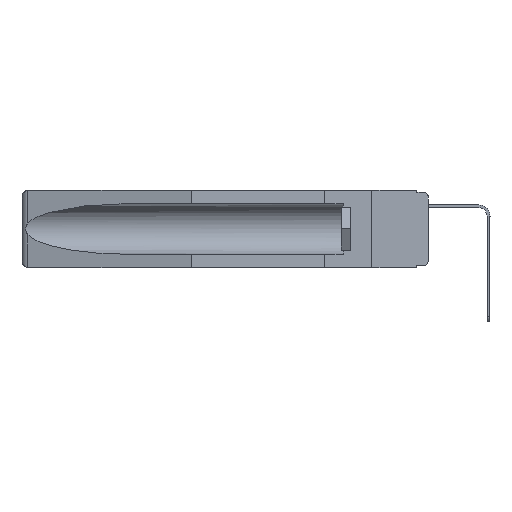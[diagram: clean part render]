
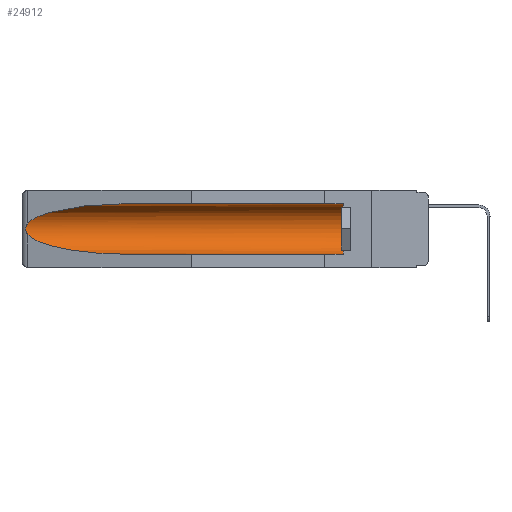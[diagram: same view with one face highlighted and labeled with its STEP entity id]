
A CAD part, left-side view. The second image highlights one B-rep face of the part: STEP entity #24912.
In plain terms, the highlighted cylindrical face has radius 2.857 mm (diameter 5.715 mm), a partial arc.
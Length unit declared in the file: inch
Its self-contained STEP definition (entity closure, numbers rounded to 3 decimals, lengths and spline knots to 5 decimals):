
#73 = CARTESIAN_POINT ( 'NONE',  ( 0.155, -0.30754, -0.059 ) ) ;
#210 = ORIENTED_EDGE ( 'NONE', *, *, #16794, .T. ) ;
#627 = VERTEX_POINT ( 'NONE', #7582 ) ;
#863 = EDGE_CURVE ( 'NONE', #627, #16626, #7154, .T. ) ;
#2396 = VERTEX_POINT ( 'NONE', #21390 ) ;
#2534 = EDGE_CURVE ( 'NONE', #627, #20455, #9218, .T. ) ;
#2753 = CARTESIAN_POINT ( 'NONE',  ( 0.2675, 1.53308, -0.17534 ) ) ;
#2929 = CARTESIAN_POINT ( 'NONE',  ( 0.155, 1.07973, -0.284 ) ) ;
#3039 = AXIS2_PLACEMENT_3D ( 'NONE', #8052, #11951, #4385 ) ;
#4385 = DIRECTION ( 'NONE',  ( 0., 0., 1. ) ) ;
#4728 = CARTESIAN_POINT ( 'NONE',  ( 0.26537, 1.52718, -0.14972 ) ) ;
#4890 = ORIENTED_EDGE ( 'NONE', *, *, #9705, .T. ) ;
#4946 = CYLINDRICAL_SURFACE ( 'NONE', #3039, 0.1125 ) ;
#5270 = VECTOR ( 'NONE', #25312, 39.37008 ) ;
#5434 = CARTESIAN_POINT ( 'NONE',  ( 0.155, 1.07973, -0.059 ) ) ;
#7154 = CIRCLE ( 'NONE', #8418, 0.1125 ) ;
#7582 = CARTESIAN_POINT ( 'NONE',  ( 0.155, 0.126, -0.284 ) ) ;
#8052 = CARTESIAN_POINT ( 'NONE',  ( 0.155, -0.30754, -0.1715 ) ) ;
#8418 = AXIS2_PLACEMENT_3D ( 'NONE', #24604, #16175, #23609 ) ;
#8905 = CARTESIAN_POINT ( 'NONE',  ( 0.21114, 1.30732, -0.284 ) ) ;
#9218 = LINE ( 'NONE', #10142, #16315 ) ;
#9551 = VERTEX_POINT ( 'NONE', #17956 ) ;
#9705 = EDGE_CURVE ( 'NONE', #9551, #20455, #12504, .T. ) ;
#10142 = CARTESIAN_POINT ( 'NONE',  ( 0.155, -0.30754, -0.284 ) ) ;
#10208 = CARTESIAN_POINT ( 'NONE',  ( 0.26597, 1.52961, -0.15275 ) ) ;
#10494 = LINE ( 'NONE', #73, #5270 ) ;
#10935 = ORIENTED_EDGE ( 'NONE', *, *, #23607, .T. ) ;
#11814 = DIRECTION ( 'NONE',  ( 0., 1., 0. ) ) ;
#11951 = DIRECTION ( 'NONE',  ( 0., 1., 0. ) ) ;
#12220 = EDGE_LOOP ( 'NONE', ( #10935, #210, #4890, #18144, #12949, #17336 ) ) ;
#12287 = CARTESIAN_POINT ( 'NONE',  ( 0.2673, 1.53269, -0.17917 ) ) ;
#12504 =( BOUNDED_CURVE ( )  B_SPLINE_CURVE ( 3, ( #22294, #20497, #8905, #2929 ),
 .UNSPECIFIED., .F., .F. ) 
 B_SPLINE_CURVE_WITH_KNOTS ( ( 4, 4 ),
 ( 0.1948, 1.5708 ),
 .UNSPECIFIED. ) 
 CURVE ( )  GEOMETRIC_REPRESENTATION_ITEM ( )  RATIONAL_B_SPLINE_CURVE ( ( 1., 0.848, 0.848, 1. ) ) 
 REPRESENTATION_ITEM ( '' )  );
#12949 = ORIENTED_EDGE ( 'NONE', *, *, #863, .T. ) ;
#13445 =( BOUNDED_CURVE ( )  B_SPLINE_CURVE ( 3, ( #5434, #17284, #23088, #23007 ),
 .UNSPECIFIED., .F., .T. ) 
 B_SPLINE_CURVE_WITH_KNOTS ( ( 4, 4 ),
 ( 4.71239, 6.08839 ),
 .UNSPECIFIED. ) 
 CURVE ( )  GEOMETRIC_REPRESENTATION_ITEM ( )  RATIONAL_B_SPLINE_CURVE ( ( 1., 0.848, 0.848, 1. ) ) 
 REPRESENTATION_ITEM ( '' )  );
#13766 = CARTESIAN_POINT ( 'NONE',  ( 0.155, 1.07973, -0.284 ) ) ;
#14045 = EDGE_CURVE ( 'NONE', #16626, #2396, #10494, .T. ) ;
#14366 = CARTESIAN_POINT ( 'NONE',  ( 0.2673, 1.5327, -0.16383 ) ) ;
#14525 = CARTESIAN_POINT ( 'NONE',  ( 0.26654, 1.53092, -0.15636 ) ) ;
#16175 = DIRECTION ( 'NONE',  ( 0., -1., 0. ) ) ;
#16315 = VECTOR ( 'NONE', #11814, 39.37008 ) ;
#16492 = CARTESIAN_POINT ( 'NONE',  ( 0.26655, 1.53094, -0.18657 ) ) ;
#16626 = VERTEX_POINT ( 'NONE', #23586 ) ;
#16794 = EDGE_CURVE ( 'NONE', #22912, #9551, #23311, .T. ) ;
#17143 = FACE_OUTER_BOUND ( 'NONE', #12220, .T. ) ;
#17284 = CARTESIAN_POINT ( 'NONE',  ( 0.21114, 1.30732, -0.059 ) ) ;
#17336 = ORIENTED_EDGE ( 'NONE', *, *, #14045, .T. ) ;
#17956 = CARTESIAN_POINT ( 'NONE',  ( 0.26537, 1.52718, -0.19328 ) ) ;
#18144 = ORIENTED_EDGE ( 'NONE', *, *, #2534, .F. ) ;
#18441 = CARTESIAN_POINT ( 'NONE',  ( 0.2675, 1.53308, -0.16763 ) ) ;
#19997 = CARTESIAN_POINT ( 'NONE',  ( 0.26597, 1.5296, -0.19026 ) ) ;
#20455 = VERTEX_POINT ( 'NONE', #13766 ) ;
#20497 = CARTESIAN_POINT ( 'NONE',  ( 0.25451, 1.48313, -0.24835 ) ) ;
#21390 = CARTESIAN_POINT ( 'NONE',  ( 0.155, 1.07973, -0.059 ) ) ;
#21958 = CARTESIAN_POINT ( 'NONE',  ( 0.26537, 1.52718, -0.19328 ) ) ;
#22294 = CARTESIAN_POINT ( 'NONE',  ( 0.26537, 1.52718, -0.19328 ) ) ;
#22912 = VERTEX_POINT ( 'NONE', #24460 ) ;
#23007 = CARTESIAN_POINT ( 'NONE',  ( 0.26537, 1.52718, -0.14972 ) ) ;
#23088 = CARTESIAN_POINT ( 'NONE',  ( 0.25451, 1.48313, -0.09465 ) ) ;
#23311 = B_SPLINE_CURVE_WITH_KNOTS ( 'NONE', 3,
 ( #4728, #10208, #14525, #14366, #18441, #2753, #12287, #16492, #19997, #21958 ),
 .UNSPECIFIED., .F., .F.,
 ( 4, 2, 2, 2, 4 ),
 ( 0., 0.00029, 0.00058, 0.00087, 0.00117 ),
 .UNSPECIFIED. ) ;
#23586 = CARTESIAN_POINT ( 'NONE',  ( 0.155, 0.126, -0.059 ) ) ;
#23607 = EDGE_CURVE ( 'NONE', #2396, #22912, #13445, .T. ) ;
#23609 = DIRECTION ( 'NONE',  ( 0., 0., 1. ) ) ;
#24460 = CARTESIAN_POINT ( 'NONE',  ( 0.26537, 1.52718, -0.14972 ) ) ;
#24604 = CARTESIAN_POINT ( 'NONE',  ( 0.155, 0.126, -0.1715 ) ) ;
#24912 = ADVANCED_FACE ( 'NONE', ( #17143 ), #4946, .F. ) ;
#25312 = DIRECTION ( 'NONE',  ( 0., 1., 0. ) ) ;
